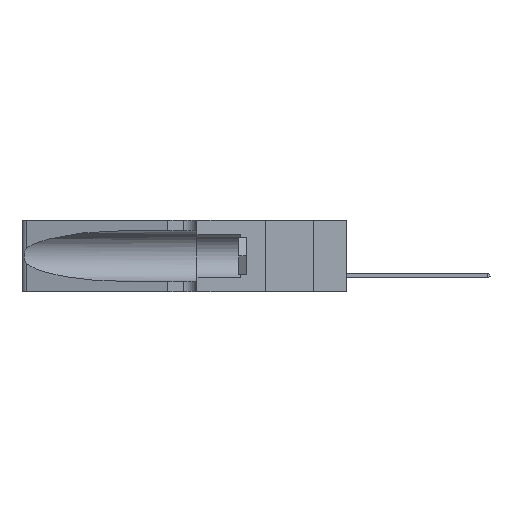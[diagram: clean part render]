
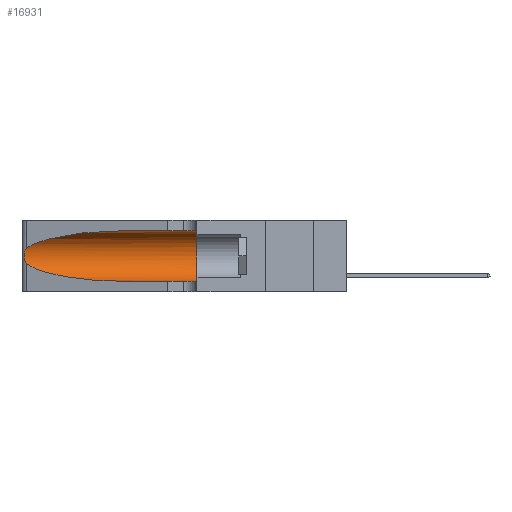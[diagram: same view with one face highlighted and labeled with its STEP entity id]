
A CAD part, left-side view. The second image highlights one B-rep face of the part: STEP entity #16931.
In plain terms, the highlighted cylindrical face has radius 3.308 mm (diameter 6.617 mm), a partial arc.
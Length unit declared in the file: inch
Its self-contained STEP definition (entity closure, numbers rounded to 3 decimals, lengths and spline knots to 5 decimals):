
#601 = CARTESIAN_POINT ( 'NONE',  ( 0.25555, 1.22994, 0.2215 ) ) ;
#618 =( BOUNDED_CURVE ( )  B_SPLINE_CURVE ( 3, ( #2816, #18561, #38063, #2956 ),
 .UNSPECIFIED., .F., .F. ) 
 B_SPLINE_CURVE_WITH_KNOTS ( ( 4, 4 ),
 ( 3.44316, 4.71239 ),
 .UNSPECIFIED. ) 
 CURVE ( )  GEOMETRIC_REPRESENTATION_ITEM ( )  RATIONAL_B_SPLINE_CURVE ( ( 1., 0.87, 0.87, 1. ) ) 
 REPRESENTATION_ITEM ( '' )  );
#643 = EDGE_CURVE ( 'NONE', #31411, #31651, #13531, .T. ) ;
#1016 = AXIS2_PLACEMENT_3D ( 'NONE', #4484, #23861, #33611 ) ;
#1458 = CARTESIAN_POINT ( 'NONE',  ( 0.26075, 1.23896, 0.19203 ) ) ;
#2816 = CARTESIAN_POINT ( 'NONE',  ( 0.25487, 1.22718, 0.14631 ) ) ;
#2956 = CARTESIAN_POINT ( 'NONE',  ( 0.1305, 0.72297, 0.05475 ) ) ;
#3571 = CARTESIAN_POINT ( 'NONE',  ( 0.1305, 0.72297, 0.31525 ) ) ;
#3867 = VERTEX_POINT ( 'NONE', #15501 ) ;
#4484 = CARTESIAN_POINT ( 'NONE',  ( 0.1305, 0.35, 0.185 ) ) ;
#4670 = EDGE_LOOP ( 'NONE', ( #28250, #20732, #38220, #20625, #12452, #37949 ) ) ;
#6634 = CARTESIAN_POINT ( 'NONE',  ( 0.25487, 1.22718, 0.22369 ) ) ;
#7313 = LINE ( 'NONE', #25515, #26277 ) ;
#7739 = VERTEX_POINT ( 'NONE', #12668 ) ;
#9661 = VERTEX_POINT ( 'NONE', #36384 ) ;
#9672 = DIRECTION ( 'NONE',  ( 0., 0., -1. ) ) ;
#10077 = DIRECTION ( 'NONE',  ( 0., -1., 0. ) ) ;
#10407 = AXIS2_PLACEMENT_3D ( 'NONE', #19261, #10077, #9672 ) ;
#10628 = CARTESIAN_POINT ( 'NONE',  ( 0.25639, 1.23186, 0.15144 ) ) ;
#11401 = DIRECTION ( 'NONE',  ( 0., -1., 0. ) ) ;
#12440 = EDGE_CURVE ( 'NONE', #7739, #28722, #7313, .T. ) ;
#12452 = ORIENTED_EDGE ( 'NONE', *, *, #26284, .F. ) ;
#12668 = CARTESIAN_POINT ( 'NONE',  ( 0.1305, 0.72297, 0.31525 ) ) ;
#12746 = FACE_OUTER_BOUND ( 'NONE', #4670, .T. ) ;
#13321 = CARTESIAN_POINT ( 'NONE',  ( 0.2373, 1.15595, 0.28018 ) ) ;
#13531 = LINE ( 'NONE', #18088, #25509 ) ;
#14111 = CARTESIAN_POINT ( 'NONE',  ( 0.25854, 1.2359, 0.20912 ) ) ;
#15501 = CARTESIAN_POINT ( 'NONE',  ( 0.25487, 1.22718, 0.22369 ) ) ;
#16094 = CARTESIAN_POINT ( 'NONE',  ( 0.1305, 0.72297, 0.05475 ) ) ;
#16931 = ADVANCED_FACE ( 'NONE', ( #12746 ), #37716, .F. ) ;
#17051 = CARTESIAN_POINT ( 'NONE',  ( 0.26075, 1.23896, 0.178 ) ) ;
#17193 = CARTESIAN_POINT ( 'NONE',  ( 0.25789, 1.23486, 0.15765 ) ) ;
#17249 =( BOUNDED_CURVE ( )  B_SPLINE_CURVE ( 3, ( #3571, #32167, #13321, #6634 ),
 .UNSPECIFIED., .F., .F. ) 
 B_SPLINE_CURVE_WITH_KNOTS ( ( 4, 4 ),
 ( 1.5708, 2.84003 ),
 .UNSPECIFIED. ) 
 CURVE ( )  GEOMETRIC_REPRESENTATION_ITEM ( )  RATIONAL_B_SPLINE_CURVE ( ( 1., 0.87, 0.87, 1. ) ) 
 REPRESENTATION_ITEM ( '' )  );
#17411 = EDGE_CURVE ( 'NONE', #7739, #3867, #17249, .T. ) ;
#17477 = CARTESIAN_POINT ( 'NONE',  ( 0.26017, 1.23833, 0.17102 ) ) ;
#18088 = CARTESIAN_POINT ( 'NONE',  ( 0.1305, 1.61858, 0.05475 ) ) ;
#18561 = CARTESIAN_POINT ( 'NONE',  ( 0.2373, 1.15595, 0.08982 ) ) ;
#18678 = DIRECTION ( 'NONE',  ( 0., -1., 0. ) ) ;
#19129 = EDGE_CURVE ( 'NONE', #9661, #31411, #618, .T. ) ;
#19261 = CARTESIAN_POINT ( 'NONE',  ( 0.1305, 1.61858, 0.185 ) ) ;
#19779 = B_SPLINE_CURVE_WITH_KNOTS ( 'NONE', 3,
 ( #32407, #601, #32543, #36548, #14111, #23738, #1458, #17051, #17477, #20395, #17193, #10628, #30188, #20093 ),
 .UNSPECIFIED., .F., .F.,
 ( 4, 2, 2, 2, 2, 2, 4 ),
 ( 0., 0.00027, 0.00053, 0.00107, 0.0016, 0.00187, 0.00214 ),
 .UNSPECIFIED. ) ;
#20093 = CARTESIAN_POINT ( 'NONE',  ( 0.25487, 1.22718, 0.14631 ) ) ;
#20395 = CARTESIAN_POINT ( 'NONE',  ( 0.25856, 1.23593, 0.16098 ) ) ;
#20625 = ORIENTED_EDGE ( 'NONE', *, *, #643, .T. ) ;
#20732 = ORIENTED_EDGE ( 'NONE', *, *, #38513, .T. ) ;
#20940 = CARTESIAN_POINT ( 'NONE',  ( 0.1305, 0.35, 0.05475 ) ) ;
#23738 = CARTESIAN_POINT ( 'NONE',  ( 0.26018, 1.23835, 0.19895 ) ) ;
#23861 = DIRECTION ( 'NONE',  ( 0., 1., 0. ) ) ;
#25509 = VECTOR ( 'NONE', #11401, 39.37008 ) ;
#25515 = CARTESIAN_POINT ( 'NONE',  ( 0.1305, 1.61858, 0.31525 ) ) ;
#26277 = VECTOR ( 'NONE', #18678, 39.37008 ) ;
#26284 = EDGE_CURVE ( 'NONE', #28722, #31651, #28271, .T. ) ;
#27513 = CARTESIAN_POINT ( 'NONE',  ( 0.1305, 0.35, 0.31525 ) ) ;
#28250 = ORIENTED_EDGE ( 'NONE', *, *, #17411, .T. ) ;
#28271 = CIRCLE ( 'NONE', #1016, 0.13025 ) ;
#28722 = VERTEX_POINT ( 'NONE', #27513 ) ;
#30188 = CARTESIAN_POINT ( 'NONE',  ( 0.25555, 1.22993, 0.14849 ) ) ;
#31411 = VERTEX_POINT ( 'NONE', #16094 ) ;
#31651 = VERTEX_POINT ( 'NONE', #20940 ) ;
#32167 = CARTESIAN_POINT ( 'NONE',  ( 0.18966, 0.96281, 0.31525 ) ) ;
#32407 = CARTESIAN_POINT ( 'NONE',  ( 0.25487, 1.22718, 0.22369 ) ) ;
#32543 = CARTESIAN_POINT ( 'NONE',  ( 0.25639, 1.23184, 0.21858 ) ) ;
#33611 = DIRECTION ( 'NONE',  ( 0., 0., 1. ) ) ;
#36384 = CARTESIAN_POINT ( 'NONE',  ( 0.25487, 1.22718, 0.14631 ) ) ;
#36548 = CARTESIAN_POINT ( 'NONE',  ( 0.25787, 1.23484, 0.2124 ) ) ;
#37716 = CYLINDRICAL_SURFACE ( 'NONE', #10407, 0.13025 ) ;
#37949 = ORIENTED_EDGE ( 'NONE', *, *, #12440, .F. ) ;
#38063 = CARTESIAN_POINT ( 'NONE',  ( 0.18966, 0.96281, 0.05475 ) ) ;
#38220 = ORIENTED_EDGE ( 'NONE', *, *, #19129, .T. ) ;
#38513 = EDGE_CURVE ( 'NONE', #3867, #9661, #19779, .T. ) ;
